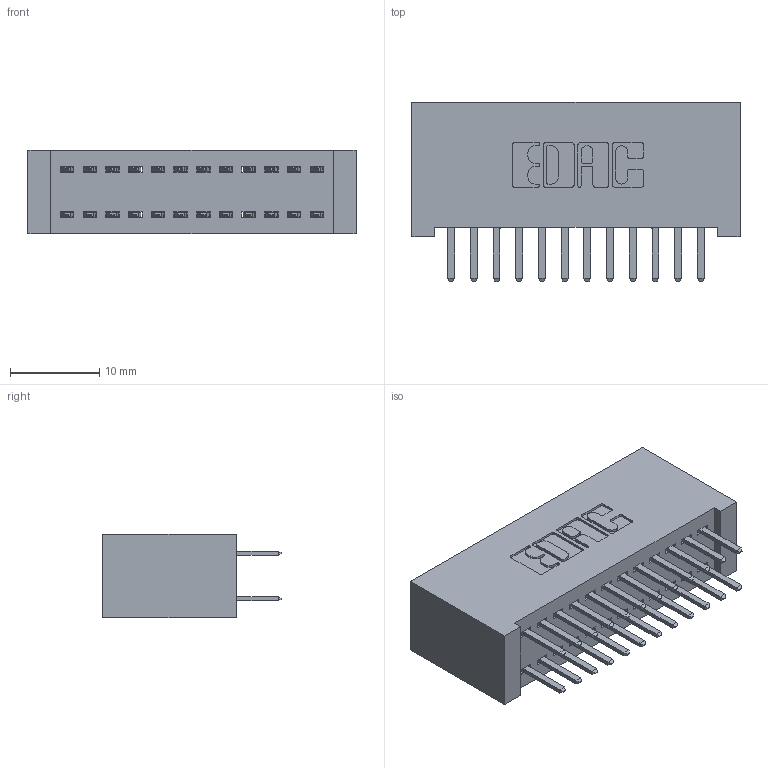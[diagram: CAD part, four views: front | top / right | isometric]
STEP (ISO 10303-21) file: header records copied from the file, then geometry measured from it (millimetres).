
FILE_DESCRIPTION (( 'STEP AP203' ), '1' );
FILE_NAME ('392-024-520-201.STEP', '2019-10-07T07:06:20', ( '' ), ( '' ), 'SwSTEP 2.0', 'SolidWorks 2016', '' );
FILE_SCHEMA (( 'CONFIG_CONTROL_DESIGN' ));
Length unit declared in the file: inch
Products named in the file (3): 345-292-001_345-293-120; 392-024-520-201; 342 Part_Lugless
Assembly tree (25 placements, depth 2):
  392-024-520-201
    342 Part_Lugless
    345-292-001_345-293-120  x24
Bounding box: 36.73 x 20.02 x 9.4 mm (x, y, z)
Volume: 3587 mm3; surface area: 5520.9 mm2
Topology: 25 solids, 25 shells, 1446 faces, 4187 edges, 2726 vertices
Faces by surface type: plane 974, cylinder 472
Entity records: 11305 total; most frequent: CARTESIAN_POINT 1918, ORIENTED_EDGE 1842, DIRECTION 1673, EDGE_CURVE 921, VECTOR 797, LINE 797, VERTEX_POINT 610, AXIS2_PLACEMENT_3D 438
